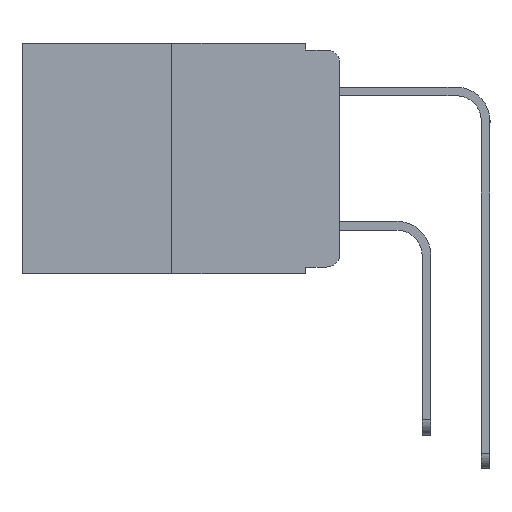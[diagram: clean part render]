
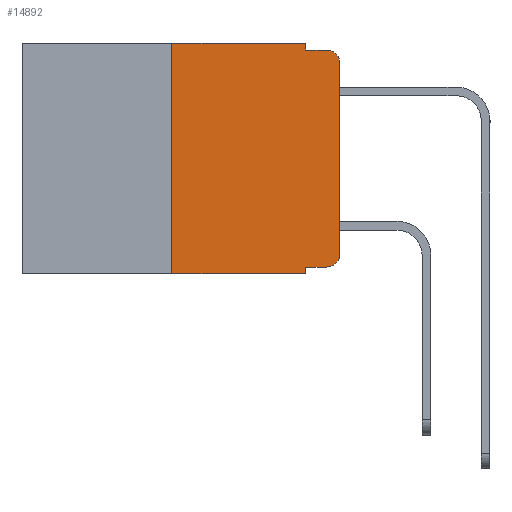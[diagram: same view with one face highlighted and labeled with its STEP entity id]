
A CAD part, left-side view. The second image highlights one B-rep face of the part: STEP entity #14892.
In plain terms, the highlighted planar face has unit normal (-1, 0, 0).
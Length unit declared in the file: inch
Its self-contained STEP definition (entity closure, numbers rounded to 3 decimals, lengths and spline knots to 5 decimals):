
#195 = VECTOR ( 'NONE', #3816, 39.37008 ) ;
#1147 = DIRECTION ( 'NONE',  ( 0., 0., -1. ) ) ;
#1178 = EDGE_CURVE ( 'NONE', #5917, #15214, #12035, .T. ) ;
#1289 = VECTOR ( 'NONE', #17414, 39.37008 ) ;
#1830 = LINE ( 'NONE', #6526, #1289 ) ;
#1862 = DIRECTION ( 'NONE',  ( 0., -1., 0. ) ) ;
#1987 = EDGE_CURVE ( 'NONE', #10898, #5459, #5088, .T. ) ;
#2566 = VECTOR ( 'NONE', #4199, 39.37008 ) ;
#2787 = CARTESIAN_POINT ( 'NONE',  ( 0., 0., 0. ) ) ;
#3075 = EDGE_CURVE ( 'NONE', #15214, #10898, #5035, .T. ) ;
#3816 = DIRECTION ( 'NONE',  ( 0., -1., 0. ) ) ;
#3865 = ORIENTED_EDGE ( 'NONE', *, *, #7066, .T. ) ;
#4115 = VERTEX_POINT ( 'NONE', #18474 ) ;
#4199 = DIRECTION ( 'NONE',  ( 0., 0., 1. ) ) ;
#4215 = EDGE_CURVE ( 'NONE', #8743, #13137, #1830, .T. ) ;
#4235 = PLANE ( 'NONE',  #10689 ) ;
#4308 = ORIENTED_EDGE ( 'NONE', *, *, #3075, .F. ) ;
#4823 = ORIENTED_EDGE ( 'NONE', *, *, #16524, .F. ) ;
#5035 = LINE ( 'NONE', #17189, #8536 ) ;
#5088 = LINE ( 'NONE', #10940, #15699 ) ;
#5089 = EDGE_CURVE ( 'NONE', #5473, #17794, #17812, .T. ) ;
#5124 = EDGE_LOOP ( 'NONE', ( #14683, #3865, #7831, #4308, #8319, #4823, #8796, #15875, #9233, #5746 ) ) ;
#5215 = CARTESIAN_POINT ( 'NONE',  ( 0., 0.051, -0.01 ) ) ;
#5382 = CARTESIAN_POINT ( 'NONE',  ( 0., 0.25, -0.343 ) ) ;
#5430 = CARTESIAN_POINT ( 'NONE',  ( 0., 0.02, -0.333 ) ) ;
#5459 = VERTEX_POINT ( 'NONE', #9351 ) ;
#5473 = VERTEX_POINT ( 'NONE', #10745 ) ;
#5746 = ORIENTED_EDGE ( 'NONE', *, *, #14802, .T. ) ;
#5762 = CARTESIAN_POINT ( 'NONE',  ( 0., 0.02, -0.03 ) ) ;
#5771 = CARTESIAN_POINT ( 'NONE',  ( 0., 0.473, 0. ) ) ;
#5917 = VERTEX_POINT ( 'NONE', #9028 ) ;
#6526 = CARTESIAN_POINT ( 'NONE',  ( 0., 0.473, -0.343 ) ) ;
#7066 = EDGE_CURVE ( 'NONE', #17794, #5459, #7387, .T. ) ;
#7240 = DIRECTION ( 'NONE',  ( 0., 0., -1. ) ) ;
#7387 = CIRCLE ( 'NONE', #16220, 0.02 ) ;
#7730 = CARTESIAN_POINT ( 'NONE',  ( 0., 0.051, 0. ) ) ;
#7831 = ORIENTED_EDGE ( 'NONE', *, *, #1987, .F. ) ;
#8319 = ORIENTED_EDGE ( 'NONE', *, *, #1178, .F. ) ;
#8431 = CARTESIAN_POINT ( 'NONE',  ( 0., 0.051, -0.343 ) ) ;
#8536 = VECTOR ( 'NONE', #14319, 39.37008 ) ;
#8591 = CARTESIAN_POINT ( 'NONE',  ( 0., 0.02, -0.313 ) ) ;
#8679 = DIRECTION ( 'NONE',  ( 0., 0., 1. ) ) ;
#8743 = VERTEX_POINT ( 'NONE', #5382 ) ;
#8796 = ORIENTED_EDGE ( 'NONE', *, *, #4215, .T. ) ;
#9028 = CARTESIAN_POINT ( 'NONE',  ( 0., 0.25, 0. ) ) ;
#9233 = ORIENTED_EDGE ( 'NONE', *, *, #13922, .T. ) ;
#9351 = CARTESIAN_POINT ( 'NONE',  ( 0., 0.02, -0.01 ) ) ;
#9580 = CIRCLE ( 'NONE', #18036, 0.02 ) ;
#10001 = DIRECTION ( 'NONE',  ( 0., 0., -1. ) ) ;
#10184 = DIRECTION ( 'NONE',  ( 1., 0., 0. ) ) ;
#10689 = AXIS2_PLACEMENT_3D ( 'NONE', #5771, #10184, #1147 ) ;
#10745 = CARTESIAN_POINT ( 'NONE',  ( 0., 0., -0.313 ) ) ;
#10833 = VECTOR ( 'NONE', #8679, 39.37008 ) ;
#10898 = VERTEX_POINT ( 'NONE', #5215 ) ;
#10940 = CARTESIAN_POINT ( 'NONE',  ( 0., 0.051, -0.01 ) ) ;
#11123 = CARTESIAN_POINT ( 'NONE',  ( 0., 0.051, -0.333 ) ) ;
#11264 = VECTOR ( 'NONE', #15839, 39.37008 ) ;
#11419 = CARTESIAN_POINT ( 'NONE',  ( 0., 0.25, 0. ) ) ;
#11641 = VECTOR ( 'NONE', #16982, 39.37008 ) ;
#11752 = LINE ( 'NONE', #11123, #195 ) ;
#12035 = LINE ( 'NONE', #13109, #11641 ) ;
#13109 = CARTESIAN_POINT ( 'NONE',  ( 0., 0.473, 0. ) ) ;
#13137 = VERTEX_POINT ( 'NONE', #8431 ) ;
#13922 = EDGE_CURVE ( 'NONE', #4115, #15579, #11752, .T. ) ;
#14319 = DIRECTION ( 'NONE',  ( 0., 0., -1. ) ) ;
#14683 = ORIENTED_EDGE ( 'NONE', *, *, #5089, .T. ) ;
#14802 = EDGE_CURVE ( 'NONE', #15579, #5473, #9580, .T. ) ;
#14892 = ADVANCED_FACE ( 'NONE', ( #15408 ), #4235, .F. ) ;
#15214 = VERTEX_POINT ( 'NONE', #17241 ) ;
#15408 = FACE_OUTER_BOUND ( 'NONE', #5124, .T. ) ;
#15440 = DIRECTION ( 'NONE',  ( -1., 0., 0. ) ) ;
#15579 = VERTEX_POINT ( 'NONE', #5430 ) ;
#15699 = VECTOR ( 'NONE', #1862, 39.37008 ) ;
#15839 = DIRECTION ( 'NONE',  ( 0., 0., -1. ) ) ;
#15875 = ORIENTED_EDGE ( 'NONE', *, *, #18248, .F. ) ;
#16220 = AXIS2_PLACEMENT_3D ( 'NONE', #5762, #15440, #7240 ) ;
#16429 = CARTESIAN_POINT ( 'NONE',  ( 0., 0., -0.03 ) ) ;
#16524 = EDGE_CURVE ( 'NONE', #8743, #5917, #18186, .T. ) ;
#16982 = DIRECTION ( 'NONE',  ( 0., -1., 0. ) ) ;
#17189 = CARTESIAN_POINT ( 'NONE',  ( 0., 0.051, 0. ) ) ;
#17241 = CARTESIAN_POINT ( 'NONE',  ( 0., 0.051, 0. ) ) ;
#17414 = DIRECTION ( 'NONE',  ( 0., -1., 0. ) ) ;
#17794 = VERTEX_POINT ( 'NONE', #16429 ) ;
#17812 = LINE ( 'NONE', #2787, #2566 ) ;
#17878 = DIRECTION ( 'NONE',  ( -1., 0., 0. ) ) ;
#18036 = AXIS2_PLACEMENT_3D ( 'NONE', #8591, #17878, #10001 ) ;
#18173 = LINE ( 'NONE', #7730, #11264 ) ;
#18186 = LINE ( 'NONE', #11419, #10833 ) ;
#18248 = EDGE_CURVE ( 'NONE', #4115, #13137, #18173, .T. ) ;
#18474 = CARTESIAN_POINT ( 'NONE',  ( 0., 0.051, -0.333 ) ) ;
